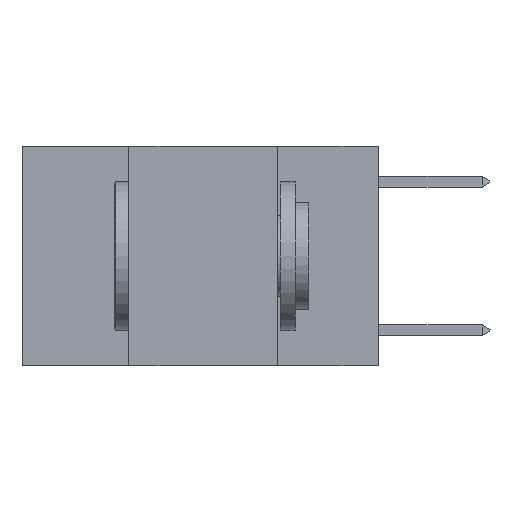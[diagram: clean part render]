
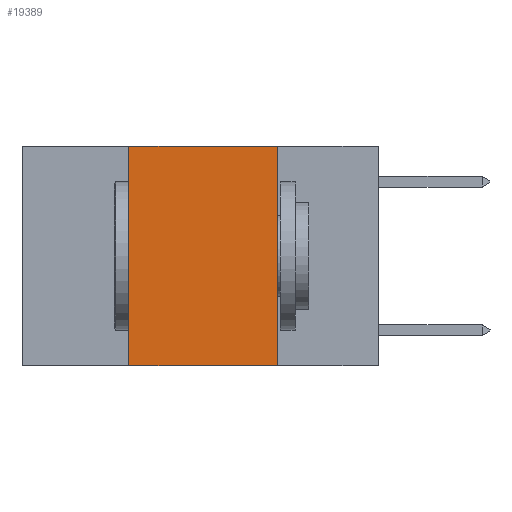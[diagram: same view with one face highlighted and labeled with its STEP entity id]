
A CAD part, left-side view. The second image highlights one B-rep face of the part: STEP entity #19389.
In plain terms, the highlighted planar face has unit normal (-1, 0, 0).
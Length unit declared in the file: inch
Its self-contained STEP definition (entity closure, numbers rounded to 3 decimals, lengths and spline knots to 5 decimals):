
#550 = CARTESIAN_POINT ( 'NONE',  ( 0., 0.42, 0. ) ) ;
#684 = DIRECTION ( 'NONE',  ( 1., 0., 0. ) ) ;
#1375 = CARTESIAN_POINT ( 'NONE',  ( 0., 0.6, 0. ) ) ;
#1625 = ORIENTED_EDGE ( 'NONE', *, *, #19660, .F. ) ;
#2178 = EDGE_CURVE ( 'NONE', #14010, #13275, #15918, .T. ) ;
#3676 = ORIENTED_EDGE ( 'NONE', *, *, #12961, .F. ) ;
#5428 = DIRECTION ( 'NONE',  ( 0., 0., -1. ) ) ;
#6184 = VECTOR ( 'NONE', #7922, 39.37008 ) ;
#7419 = VECTOR ( 'NONE', #9768, 39.37008 ) ;
#7921 = CARTESIAN_POINT ( 'NONE',  ( 0., 0.42, 0. ) ) ;
#7922 = DIRECTION ( 'NONE',  ( 0., -1., 0. ) ) ;
#8754 = EDGE_LOOP ( 'NONE', ( #12672, #1625, #3676, #10185 ) ) ;
#9487 = LINE ( 'NONE', #1375, #6184 ) ;
#9622 = CARTESIAN_POINT ( 'NONE',  ( 0., 0.42, -0.37 ) ) ;
#9768 = DIRECTION ( 'NONE',  ( 0., -1., 0. ) ) ;
#10185 = ORIENTED_EDGE ( 'NONE', *, *, #2178, .T. ) ;
#10414 = CARTESIAN_POINT ( 'NONE',  ( 0., 0.6, 0. ) ) ;
#11403 = VERTEX_POINT ( 'NONE', #7921 ) ;
#12039 = DIRECTION ( 'NONE',  ( 0., 0., -1. ) ) ;
#12057 = LINE ( 'NONE', #550, #19815 ) ;
#12672 = ORIENTED_EDGE ( 'NONE', *, *, #15507, .F. ) ;
#12743 = CARTESIAN_POINT ( 'NONE',  ( 0., 0.17, -0.37 ) ) ;
#12961 = EDGE_CURVE ( 'NONE', #14010, #11403, #12057, .T. ) ;
#13275 = VERTEX_POINT ( 'NONE', #12743 ) ;
#13396 = VECTOR ( 'NONE', #5428, 39.37008 ) ;
#13993 = FACE_OUTER_BOUND ( 'NONE', #8754, .T. ) ;
#14010 = VERTEX_POINT ( 'NONE', #9622 ) ;
#15507 = EDGE_CURVE ( 'NONE', #16651, #13275, #17546, .T. ) ;
#15918 = LINE ( 'NONE', #16090, #7419 ) ;
#16090 = CARTESIAN_POINT ( 'NONE',  ( 0., 0.6, -0.37 ) ) ;
#16651 = VERTEX_POINT ( 'NONE', #17785 ) ;
#16695 = PLANE ( 'NONE',  #18917 ) ;
#17546 = LINE ( 'NONE', #19571, #13396 ) ;
#17785 = CARTESIAN_POINT ( 'NONE',  ( 0., 0.17, 0. ) ) ;
#18149 = DIRECTION ( 'NONE',  ( 0., 0., 1. ) ) ;
#18917 = AXIS2_PLACEMENT_3D ( 'NONE', #10414, #684, #12039 ) ;
#19389 = ADVANCED_FACE ( 'NONE', ( #13993 ), #16695, .F. ) ;
#19571 = CARTESIAN_POINT ( 'NONE',  ( 0., 0.17, 0. ) ) ;
#19660 = EDGE_CURVE ( 'NONE', #11403, #16651, #9487, .T. ) ;
#19815 = VECTOR ( 'NONE', #18149, 39.37008 ) ;
